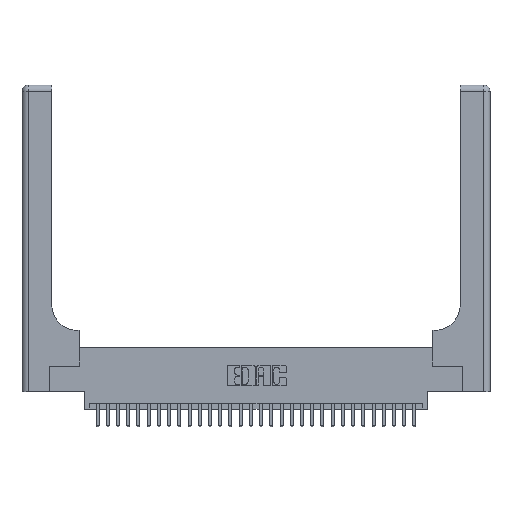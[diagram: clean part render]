
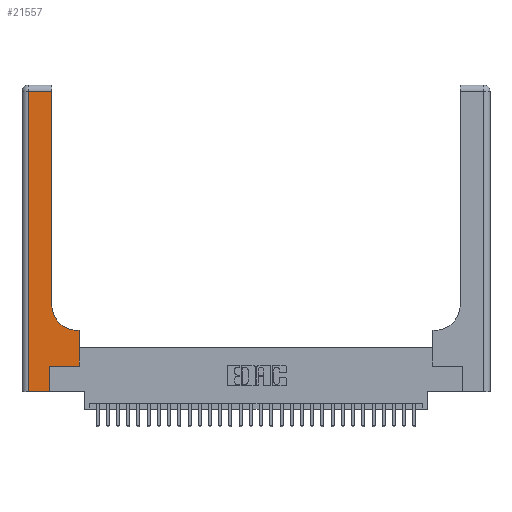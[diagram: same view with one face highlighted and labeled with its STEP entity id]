
A CAD part, top view. The second image highlights one B-rep face of the part: STEP entity #21557.
In plain terms, the highlighted planar face has unit normal (0, 0, 1).
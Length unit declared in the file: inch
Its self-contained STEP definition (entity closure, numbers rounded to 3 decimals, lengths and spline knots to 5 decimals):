
#383 = EDGE_CURVE ( 'NONE', #24605, #1269, #19570, .T. ) ;
#703 = DIRECTION ( 'NONE',  ( 0., 1., 0. ) ) ;
#753 = CARTESIAN_POINT ( 'NONE',  ( 0.06, 3., 0.37 ) ) ;
#755 = VECTOR ( 'NONE', #3295, 39.37008 ) ;
#1269 = VERTEX_POINT ( 'NONE', #29983 ) ;
#1618 = DIRECTION ( 'NONE',  ( 0., 0., -1. ) ) ;
#2045 = EDGE_LOOP ( 'NONE', ( #28673, #25662, #5165, #11143, #20354, #16176, #29034, #29606, #10183 ) ) ;
#2458 = CARTESIAN_POINT ( 'NONE',  ( 0.269, 0.25, 0.37 ) ) ;
#2505 = DIRECTION ( 'NONE',  ( -1., 0., 0. ) ) ;
#2542 = CARTESIAN_POINT ( 'NONE',  ( 0.2915, 0.6, 0.37 ) ) ;
#2558 = CARTESIAN_POINT ( 'NONE',  ( 0.06, 0., 0.37 ) ) ;
#2844 = VECTOR ( 'NONE', #15126, 39.37008 ) ;
#3295 = DIRECTION ( 'NONE',  ( 0., -1., 0. ) ) ;
#3639 = LINE ( 'NONE', #12645, #2844 ) ;
#4574 = VERTEX_POINT ( 'NONE', #21352 ) ;
#5165 = ORIENTED_EDGE ( 'NONE', *, *, #26478, .T. ) ;
#5183 = CIRCLE ( 'NONE', #24571, 0.25 ) ;
#5679 = LINE ( 'NONE', #20287, #11664 ) ;
#5986 = DIRECTION ( 'NONE',  ( 0., 0., -1. ) ) ;
#6015 = VERTEX_POINT ( 'NONE', #9541 ) ;
#6599 = VERTEX_POINT ( 'NONE', #9058 ) ;
#6632 = LINE ( 'NONE', #28774, #12630 ) ;
#7482 = VECTOR ( 'NONE', #703, 39.37008 ) ;
#7940 = DIRECTION ( 'NONE',  ( 0., 1., 0. ) ) ;
#8553 = LINE ( 'NONE', #13330, #7482 ) ;
#9058 = CARTESIAN_POINT ( 'NONE',  ( 0.2915, 0.85, 0.37 ) ) ;
#9084 = EDGE_CURVE ( 'NONE', #31191, #27899, #29361, .T. ) ;
#9541 = CARTESIAN_POINT ( 'NONE',  ( 0.269, 0.25, 0.37 ) ) ;
#9979 = CARTESIAN_POINT ( 'NONE',  ( 0.2915, 2.94, 0.37 ) ) ;
#10183 = ORIENTED_EDGE ( 'NONE', *, *, #31628, .T. ) ;
#10812 = EDGE_CURVE ( 'NONE', #6015, #25373, #12176, .T. ) ;
#11143 = ORIENTED_EDGE ( 'NONE', *, *, #15873, .T. ) ;
#11158 = CARTESIAN_POINT ( 'NONE',  ( 0.06, 2.94, 0.37 ) ) ;
#11664 = VECTOR ( 'NONE', #7940, 39.37008 ) ;
#12018 = CARTESIAN_POINT ( 'NONE',  ( 0., 2.94, 0.37 ) ) ;
#12176 = LINE ( 'NONE', #2458, #23581 ) ;
#12630 = VECTOR ( 'NONE', #14292, 39.37008 ) ;
#12645 = CARTESIAN_POINT ( 'NONE',  ( 0.2915, 3., 0.37 ) ) ;
#13330 = CARTESIAN_POINT ( 'NONE',  ( 0.269, 0., 0.37 ) ) ;
#14292 = DIRECTION ( 'NONE',  ( 1., 0., 0. ) ) ;
#14498 = DIRECTION ( 'NONE',  ( -1., 0., 0. ) ) ;
#15126 = DIRECTION ( 'NONE',  ( 0., 1., 0. ) ) ;
#15873 = EDGE_CURVE ( 'NONE', #22539, #4574, #6632, .T. ) ;
#15997 = CARTESIAN_POINT ( 'NONE',  ( 0., 3., 0.37 ) ) ;
#16176 = ORIENTED_EDGE ( 'NONE', *, *, #10812, .T. ) ;
#16685 = CARTESIAN_POINT ( 'NONE',  ( 0.5415, 0.85, 0.37 ) ) ;
#17472 = DIRECTION ( 'NONE',  ( 1., 0., 0. ) ) ;
#18875 = EDGE_CURVE ( 'NONE', #25373, #24605, #5679, .T. ) ;
#19117 = DIRECTION ( 'NONE',  ( 1., 0., 0. ) ) ;
#19570 = LINE ( 'NONE', #2542, #31635 ) ;
#20287 = CARTESIAN_POINT ( 'NONE',  ( 0.5585, 0.25, 0.37 ) ) ;
#20354 = ORIENTED_EDGE ( 'NONE', *, *, #25229, .T. ) ;
#20659 = LINE ( 'NONE', #753, #755 ) ;
#20872 = PLANE ( 'NONE',  #23762 ) ;
#21183 = CARTESIAN_POINT ( 'NONE',  ( 0.5585, 0.25, 0.37 ) ) ;
#21352 = CARTESIAN_POINT ( 'NONE',  ( 0.269, 0., 0.37 ) ) ;
#21557 = ADVANCED_FACE ( 'NONE', ( #28387 ), #20872, .F. ) ;
#22539 = VERTEX_POINT ( 'NONE', #2558 ) ;
#23311 = DIRECTION ( 'NONE',  ( -1., 0., 0. ) ) ;
#23581 = VECTOR ( 'NONE', #17472, 39.37008 ) ;
#23762 = AXIS2_PLACEMENT_3D ( 'NONE', #15997, #5986, #23311 ) ;
#24571 = AXIS2_PLACEMENT_3D ( 'NONE', #16685, #1618, #19117 ) ;
#24605 = VERTEX_POINT ( 'NONE', #29993 ) ;
#25229 = EDGE_CURVE ( 'NONE', #4574, #6015, #8553, .T. ) ;
#25373 = VERTEX_POINT ( 'NONE', #21183 ) ;
#25662 = ORIENTED_EDGE ( 'NONE', *, *, #9084, .T. ) ;
#26478 = EDGE_CURVE ( 'NONE', #27899, #22539, #20659, .T. ) ;
#27899 = VERTEX_POINT ( 'NONE', #11158 ) ;
#28387 = FACE_OUTER_BOUND ( 'NONE', #2045, .T. ) ;
#28590 = VECTOR ( 'NONE', #14498, 39.37008 ) ;
#28673 = ORIENTED_EDGE ( 'NONE', *, *, #31248, .T. ) ;
#28774 = CARTESIAN_POINT ( 'NONE',  ( 0., 0., 0.37 ) ) ;
#29034 = ORIENTED_EDGE ( 'NONE', *, *, #18875, .T. ) ;
#29361 = LINE ( 'NONE', #12018, #28590 ) ;
#29606 = ORIENTED_EDGE ( 'NONE', *, *, #383, .T. ) ;
#29983 = CARTESIAN_POINT ( 'NONE',  ( 0.5415, 0.6, 0.37 ) ) ;
#29993 = CARTESIAN_POINT ( 'NONE',  ( 0.5585, 0.6, 0.37 ) ) ;
#31191 = VERTEX_POINT ( 'NONE', #9979 ) ;
#31248 = EDGE_CURVE ( 'NONE', #6599, #31191, #3639, .T. ) ;
#31628 = EDGE_CURVE ( 'NONE', #1269, #6599, #5183, .T. ) ;
#31635 = VECTOR ( 'NONE', #2505, 39.37008 ) ;
